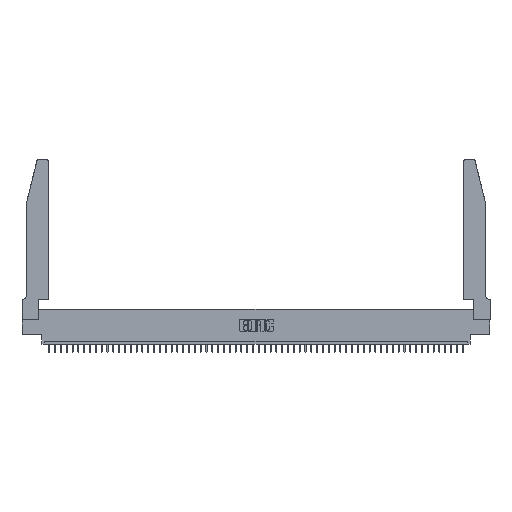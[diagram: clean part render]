
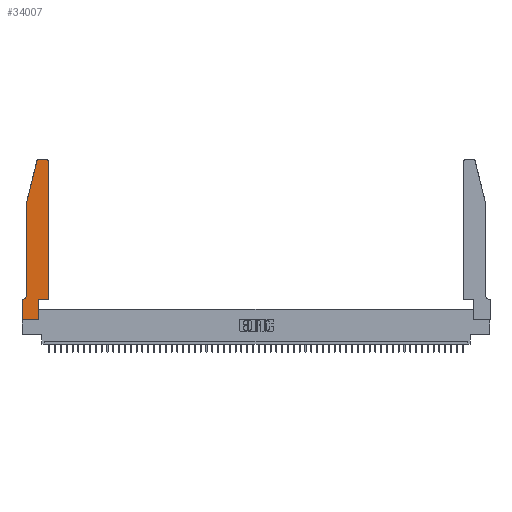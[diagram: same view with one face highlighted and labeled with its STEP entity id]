
A CAD part, top view. The second image highlights one B-rep face of the part: STEP entity #34007.
In plain terms, the highlighted planar face has unit normal (0, 0, 1).
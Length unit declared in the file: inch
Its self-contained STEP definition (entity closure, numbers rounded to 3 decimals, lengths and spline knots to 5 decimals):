
#211 = VECTOR ( 'NONE', #26446, 39.37008 ) ;
#1036 = VECTOR ( 'NONE', #7312, 39.37008 ) ;
#1504 = EDGE_CURVE ( 'NONE', #11268, #12855, #28388, .T. ) ;
#2049 = ORIENTED_EDGE ( 'NONE', *, *, #14018, .T. ) ;
#2180 = DIRECTION ( 'NONE',  ( 1., 0., 0. ) ) ;
#2298 = EDGE_LOOP ( 'NONE', ( #27936, #50846, #2049, #46037, #14651, #51019, #35232, #12668, #22904, #19171, #47223, #37639 ) ) ;
#3484 = DIRECTION ( 'NONE',  ( 0., -1., 0. ) ) ;
#4545 = DIRECTION ( 'NONE',  ( 0., 0., 1. ) ) ;
#4793 = VECTOR ( 'NONE', #37610, 39.37008 ) ;
#6867 = VERTEX_POINT ( 'NONE', #25809 ) ;
#7312 = DIRECTION ( 'NONE',  ( -1., 0., 0. ) ) ;
#9886 = LINE ( 'NONE', #15189, #32189 ) ;
#11268 = VERTEX_POINT ( 'NONE', #20355 ) ;
#11537 = CARTESIAN_POINT ( 'NONE',  ( 0.0755, 0.35, 0.37 ) ) ;
#11812 = CARTESIAN_POINT ( 'NONE',  ( 0.4505, 0.35, 0.37 ) ) ;
#11834 = EDGE_CURVE ( 'NONE', #34991, #29945, #15188, .T. ) ;
#12080 = LINE ( 'NONE', #11812, #41135 ) ;
#12668 = ORIENTED_EDGE ( 'NONE', *, *, #26882, .T. ) ;
#12855 = VERTEX_POINT ( 'NONE', #39807 ) ;
#14018 = EDGE_CURVE ( 'NONE', #46279, #36176, #9886, .T. ) ;
#14378 = DIRECTION ( 'NONE',  ( 1., 0., 0. ) ) ;
#14651 = ORIENTED_EDGE ( 'NONE', *, *, #30024, .T. ) ;
#14976 = VECTOR ( 'NONE', #14378, 39.37008 ) ;
#14993 = VECTOR ( 'NONE', #3484, 39.37008 ) ;
#15188 = CIRCLE ( 'NONE', #22231, 0.03 ) ;
#15189 = CARTESIAN_POINT ( 'NONE',  ( 0.0755, 2., 0.37 ) ) ;
#15287 = FACE_OUTER_BOUND ( 'NONE', #2298, .T. ) ;
#15585 = DIRECTION ( 'NONE',  ( 0., 0., 1. ) ) ;
#17528 = CARTESIAN_POINT ( 'NONE',  ( 0.4505, 2.72, 0.37 ) ) ;
#18308 = CARTESIAN_POINT ( 'NONE',  ( 0.4505, 0.35, 0.37 ) ) ;
#19171 = ORIENTED_EDGE ( 'NONE', *, *, #40650, .T. ) ;
#19507 = CARTESIAN_POINT ( 'NONE',  ( 0.0755, 0.42, 0.37 ) ) ;
#19947 = DIRECTION ( 'NONE',  ( 1., 0., 0. ) ) ;
#20355 = CARTESIAN_POINT ( 'NONE',  ( 0., 0.35, 0.37 ) ) ;
#22231 = AXIS2_PLACEMENT_3D ( 'NONE', #39397, #36333, #35741 ) ;
#22442 = DIRECTION ( 'NONE',  ( 1., 0., 0. ) ) ;
#22648 = LINE ( 'NONE', #39907, #39548 ) ;
#22904 = ORIENTED_EDGE ( 'NONE', *, *, #27507, .T. ) ;
#23589 = LINE ( 'NONE', #45042, #48288 ) ;
#24331 = CARTESIAN_POINT ( 'NONE',  ( 0.0755, 2., 0.37 ) ) ;
#24562 = CARTESIAN_POINT ( 'NONE',  ( 0.0055, 0.42, 0.37 ) ) ;
#25809 = CARTESIAN_POINT ( 'NONE',  ( 0.4505, 0.35, 0.37 ) ) ;
#25922 = EDGE_CURVE ( 'NONE', #6867, #34991, #12080, .T. ) ;
#26446 = DIRECTION ( 'NONE',  ( 0., 1., 0. ) ) ;
#26882 = EDGE_CURVE ( 'NONE', #12855, #34608, #23589, .T. ) ;
#26913 = EDGE_CURVE ( 'NONE', #54836, #11268, #32768, .T. ) ;
#27020 = CARTESIAN_POINT ( 'NONE',  ( 0.2865, 0.35, 0.37 ) ) ;
#27219 = AXIS2_PLACEMENT_3D ( 'NONE', #24562, #36527, #52191 ) ;
#27507 = EDGE_CURVE ( 'NONE', #34608, #40664, #52815, .T. ) ;
#27936 = ORIENTED_EDGE ( 'NONE', *, *, #29107, .T. ) ;
#28183 = PLANE ( 'NONE',  #48716 ) ;
#28388 = LINE ( 'NONE', #32268, #14993 ) ;
#28945 = CARTESIAN_POINT ( 'NONE',  ( 0.0055, 0.35, 0.37 ) ) ;
#29107 = EDGE_CURVE ( 'NONE', #29945, #34214, #46536, .T. ) ;
#29945 = VERTEX_POINT ( 'NONE', #34647 ) ;
#30024 = EDGE_CURVE ( 'NONE', #54435, #54836, #35152, .T. ) ;
#32189 = VECTOR ( 'NONE', #35824, 39.37008 ) ;
#32268 = CARTESIAN_POINT ( 'NONE',  ( 0., 0., 0.37 ) ) ;
#32768 = LINE ( 'NONE', #11537, #1036 ) ;
#34007 = ADVANCED_FACE ( 'NONE', ( #15287 ), #28183, .T. ) ;
#34214 = VERTEX_POINT ( 'NONE', #38405 ) ;
#34608 = VERTEX_POINT ( 'NONE', #38486 ) ;
#34647 = CARTESIAN_POINT ( 'NONE',  ( 0.4205, 2.75, 0.37 ) ) ;
#34991 = VERTEX_POINT ( 'NONE', #17528 ) ;
#35152 = CIRCLE ( 'NONE', #27219, 0.07 ) ;
#35232 = ORIENTED_EDGE ( 'NONE', *, *, #1504, .T. ) ;
#35741 = DIRECTION ( 'NONE',  ( 1., 0., 0. ) ) ;
#35824 = DIRECTION ( 'NONE',  ( -0.239, -0.971, 0. ) ) ;
#36176 = VERTEX_POINT ( 'NONE', #24331 ) ;
#36333 = DIRECTION ( 'NONE',  ( 0., 0., 1. ) ) ;
#36527 = DIRECTION ( 'NONE',  ( 0., 0., -1. ) ) ;
#37610 = DIRECTION ( 'NONE',  ( -1., 0., 0. ) ) ;
#37639 = ORIENTED_EDGE ( 'NONE', *, *, #11834, .T. ) ;
#38405 = CARTESIAN_POINT ( 'NONE',  ( 0.284, 2.75, 0.37 ) ) ;
#38486 = CARTESIAN_POINT ( 'NONE',  ( 0.2865, 0., 0.37 ) ) ;
#38602 = AXIS2_PLACEMENT_3D ( 'NONE', #46987, #4545, #22442 ) ;
#39397 = CARTESIAN_POINT ( 'NONE',  ( 0.4205, 2.72, 0.37 ) ) ;
#39548 = VECTOR ( 'NONE', #44384, 39.37008 ) ;
#39807 = CARTESIAN_POINT ( 'NONE',  ( 0., 0., 0.37 ) ) ;
#39907 = CARTESIAN_POINT ( 'NONE',  ( 0.0755, 2., 0.37 ) ) ;
#40650 = EDGE_CURVE ( 'NONE', #40664, #6867, #53128, .T. ) ;
#40664 = VERTEX_POINT ( 'NONE', #27020 ) ;
#41135 = VECTOR ( 'NONE', #41948, 39.37008 ) ;
#41948 = DIRECTION ( 'NONE',  ( 0., 1., 0. ) ) ;
#44174 = CARTESIAN_POINT ( 'NONE',  ( 0.25487, 2.72718, 0.37 ) ) ;
#44384 = DIRECTION ( 'NONE',  ( 0., -1., 0. ) ) ;
#45042 = CARTESIAN_POINT ( 'NONE',  ( 0., 0., 0.37 ) ) ;
#45153 = CARTESIAN_POINT ( 'NONE',  ( 0., 0.35, 0.37 ) ) ;
#45751 = CIRCLE ( 'NONE', #38602, 0.03 ) ;
#46037 = ORIENTED_EDGE ( 'NONE', *, *, #49815, .T. ) ;
#46279 = VERTEX_POINT ( 'NONE', #44174 ) ;
#46536 = LINE ( 'NONE', #54316, #4793 ) ;
#46987 = CARTESIAN_POINT ( 'NONE',  ( 0.284, 2.72, 0.37 ) ) ;
#47223 = ORIENTED_EDGE ( 'NONE', *, *, #25922, .T. ) ;
#47576 = CARTESIAN_POINT ( 'NONE',  ( 0.2865, 0.35, 0.37 ) ) ;
#48288 = VECTOR ( 'NONE', #19947, 39.37008 ) ;
#48716 = AXIS2_PLACEMENT_3D ( 'NONE', #45153, #15585, #2180 ) ;
#49815 = EDGE_CURVE ( 'NONE', #36176, #54435, #22648, .T. ) ;
#50846 = ORIENTED_EDGE ( 'NONE', *, *, #54272, .T. ) ;
#51019 = ORIENTED_EDGE ( 'NONE', *, *, #26913, .T. ) ;
#52191 = DIRECTION ( 'NONE',  ( -1., 0., 0. ) ) ;
#52815 = LINE ( 'NONE', #47576, #211 ) ;
#53128 = LINE ( 'NONE', #18308, #14976 ) ;
#54272 = EDGE_CURVE ( 'NONE', #34214, #46279, #45751, .T. ) ;
#54316 = CARTESIAN_POINT ( 'NONE',  ( 0.2605, 2.75, 0.37 ) ) ;
#54435 = VERTEX_POINT ( 'NONE', #19507 ) ;
#54836 = VERTEX_POINT ( 'NONE', #28945 ) ;
